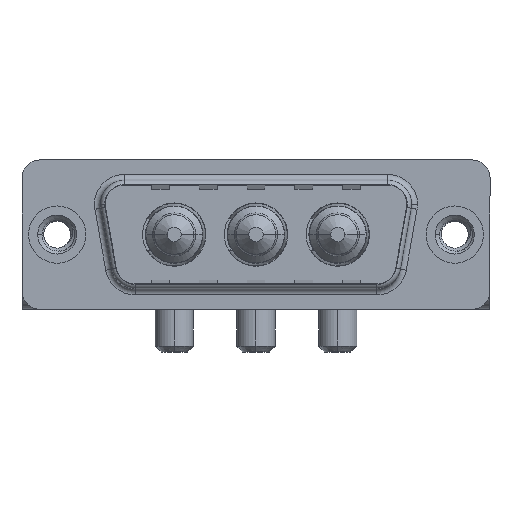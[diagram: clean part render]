
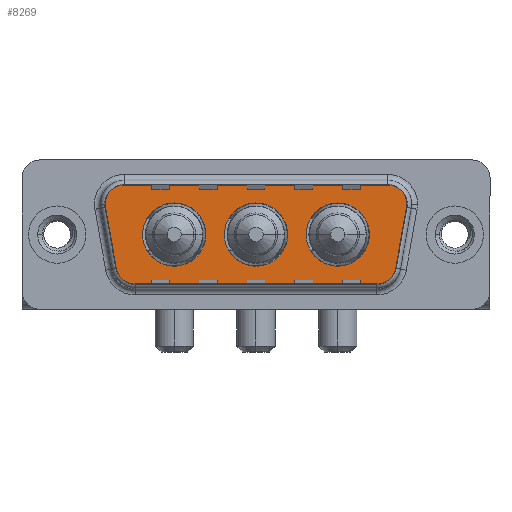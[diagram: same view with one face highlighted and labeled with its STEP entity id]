
A CAD part, top view. The second image highlights one B-rep face of the part: STEP entity #8269.
In plain terms, the highlighted planar face has unit normal (0, 0, 1).
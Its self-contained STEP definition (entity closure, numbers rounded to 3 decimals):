
#86 = VECTOR ( 'NONE', #13259, 1000. ) ;
#158 = CARTESIAN_POINT ( 'NONE',  ( 16.65, 0., 0. ) ) ;
#438 = CARTESIAN_POINT ( 'NONE',  ( 9.8, 0., 0. ) ) ;
#579 = ORIENTED_EDGE ( 'NONE', *, *, #2384, .F. ) ;
#604 = CARTESIAN_POINT ( 'NONE',  ( 5.411, 2.9, 0. ) ) ;
#606 = EDGE_CURVE ( 'NONE', #11019, #8683, #7015, .T. ) ;
#707 = ORIENTED_EDGE ( 'NONE', *, *, #3189, .T. ) ;
#709 = DIRECTION ( 'NONE',  ( 1., 0., 0. ) ) ;
#790 = DIRECTION ( 'NONE',  ( 0., 0., 1. ) ) ;
#871 = ORIENTED_EDGE ( 'NONE', *, *, #606, .T. ) ;
#988 = EDGE_CURVE ( 'NONE', #10043, #11019, #12778, .T. ) ;
#1168 = AXIS2_PLACEMENT_3D ( 'NONE', #10841, #5732, #5518 ) ;
#1506 = CARTESIAN_POINT ( 'NONE',  ( 29.889, 2.9, 0. ) ) ;
#1746 = FACE_BOUND ( 'NONE', #6988, .T. ) ;
#1797 = CARTESIAN_POINT ( 'NONE',  ( 29.859, 2.553, 0. ) ) ;
#1810 = EDGE_CURVE ( 'NONE', #2459, #10043, #4019, .T. ) ;
#1929 = VERTEX_POINT ( 'NONE', #11350 ) ;
#1930 = ORIENTED_EDGE ( 'NONE', *, *, #6689, .F. ) ;
#2007 = AXIS2_PLACEMENT_3D ( 'NONE', #6877, #3414, #4720 ) ;
#2245 = AXIS2_PLACEMENT_3D ( 'NONE', #158, #6421, #7410 ) ;
#2384 = EDGE_CURVE ( 'NONE', #12608, #10893, #13707, .T. ) ;
#2459 = VERTEX_POINT ( 'NONE', #3282 ) ;
#2910 = CIRCLE ( 'NONE', #2007, 2. ) ;
#3064 = DIRECTION ( 'NONE',  ( 0.174, -0.985, 0. ) ) ;
#3143 = EDGE_CURVE ( 'NONE', #6849, #7080, #2910, .T. ) ;
#3158 = DIRECTION ( 'NONE',  ( 0., 0., 1. ) ) ;
#3189 = EDGE_CURVE ( 'NONE', #7080, #8684, #8976, .T. ) ;
#3282 = CARTESIAN_POINT ( 'NONE',  ( 5.411, 4.9, 0. ) ) ;
#3364 = CIRCLE ( 'NONE', #13649, 2. ) ;
#3414 = DIRECTION ( 'NONE',  ( 0., 0., 1. ) ) ;
#3438 = ORIENTED_EDGE ( 'NONE', *, *, #8021, .T. ) ;
#3550 = ORIENTED_EDGE ( 'NONE', *, *, #9644, .F. ) ;
#3676 = EDGE_CURVE ( 'NONE', #13071, #8452, #9568, .T. ) ;
#3910 = VERTEX_POINT ( 'NONE', #6340 ) ;
#4019 = CIRCLE ( 'NONE', #13632, 2. ) ;
#4056 = DIRECTION ( 'NONE',  ( 0., 0., 1. ) ) ;
#4114 = CARTESIAN_POINT ( 'NONE',  ( 3.441, 2.553, 0. ) ) ;
#4203 = DIRECTION ( 'NONE',  ( -1., 0., 0. ) ) ;
#4568 = AXIS2_PLACEMENT_3D ( 'NONE', #6428, #3158, #4203 ) ;
#4661 = CARTESIAN_POINT ( 'NONE',  ( 20.85, 0., 0. ) ) ;
#4696 = DIRECTION ( 'NONE',  ( 0., 0., 1. ) ) ;
#4701 = DIRECTION ( 'NONE',  ( 1., 0., 0. ) ) ;
#4717 = CIRCLE ( 'NONE', #8948, 2.65 ) ;
#4720 = DIRECTION ( 'NONE',  ( 1., 0., 0. ) ) ;
#4723 = CIRCLE ( 'NONE', #10959, 2.65 ) ;
#4849 = EDGE_CURVE ( 'NONE', #12040, #1929, #6034, .T. ) ;
#4884 = CARTESIAN_POINT ( 'NONE',  ( 12.45, 0., 0. ) ) ;
#4943 = AXIS2_PLACEMENT_3D ( 'NONE', #6475, #9352, #13788 ) ;
#4944 = CARTESIAN_POINT ( 'NONE',  ( 6.434, -4.9, 0. ) ) ;
#5052 = DIRECTION ( 'NONE',  ( 1., 0., 0. ) ) ;
#5430 = EDGE_CURVE ( 'NONE', #8452, #13071, #13432, .T. ) ;
#5518 = DIRECTION ( 'NONE',  ( -1., 0., 0. ) ) ;
#5732 = DIRECTION ( 'NONE',  ( 0., 0., 1. ) ) ;
#5770 = DIRECTION ( 'NONE',  ( -1., 0., 0. ) ) ;
#5779 = VECTOR ( 'NONE', #8898, 1000. ) ;
#5873 = AXIS2_PLACEMENT_3D ( 'NONE', #13583, #790, #5052 ) ;
#5900 = LINE ( 'NONE', #10170, #5779 ) ;
#5956 = CARTESIAN_POINT ( 'NONE',  ( 14., 0., 0. ) ) ;
#6034 = CIRCLE ( 'NONE', #2245, 2.65 ) ;
#6064 = FACE_BOUND ( 'NONE', #9655, .T. ) ;
#6129 = CARTESIAN_POINT ( 'NONE',  ( 28.836, -3.247, 0. ) ) ;
#6251 = EDGE_CURVE ( 'NONE', #9187, #3910, #3364, .T. ) ;
#6340 = CARTESIAN_POINT ( 'NONE',  ( 27.889, 4.9, 0. ) ) ;
#6421 = DIRECTION ( 'NONE',  ( 0., 0., 1. ) ) ;
#6428 = CARTESIAN_POINT ( 'NONE',  ( 6.434, -2.9, 0. ) ) ;
#6475 = CARTESIAN_POINT ( 'NONE',  ( 23.5, 0., 0. ) ) ;
#6567 = ORIENTED_EDGE ( 'NONE', *, *, #9221, .T. ) ;
#6689 = EDGE_CURVE ( 'NONE', #1929, #12040, #4717, .T. ) ;
#6797 = DIRECTION ( 'NONE',  ( 0., 0., 1. ) ) ;
#6849 = VERTEX_POINT ( 'NONE', #10753 ) ;
#6877 = CARTESIAN_POINT ( 'NONE',  ( 26.866, -2.9, 0. ) ) ;
#6977 = CIRCLE ( 'NONE', #1168, 2. ) ;
#6988 = EDGE_LOOP ( 'NONE', ( #10766, #7136 ) ) ;
#7015 = CIRCLE ( 'NONE', #4568, 2. ) ;
#7080 = VERTEX_POINT ( 'NONE', #6129 ) ;
#7136 = ORIENTED_EDGE ( 'NONE', *, *, #5430, .F. ) ;
#7196 = AXIS2_PLACEMENT_3D ( 'NONE', #8430, #13775, #12579 ) ;
#7217 = ORIENTED_EDGE ( 'NONE', *, *, #4849, .F. ) ;
#7410 = DIRECTION ( 'NONE',  ( 1., 0., 0. ) ) ;
#7511 = ORIENTED_EDGE ( 'NONE', *, *, #3143, .T. ) ;
#7791 = DIRECTION ( 'NONE',  ( 0., 0., 1. ) ) ;
#8011 = CARTESIAN_POINT ( 'NONE',  ( 4.464, -3.247, 0. ) ) ;
#8021 = EDGE_CURVE ( 'NONE', #8684, #9187, #6977, .T. ) ;
#8026 = CARTESIAN_POINT ( 'NONE',  ( 3.441, 2.553, 0. ) ) ;
#8190 = EDGE_LOOP ( 'NONE', ( #1930, #7217 ) ) ;
#8258 = ORIENTED_EDGE ( 'NONE', *, *, #988, .T. ) ;
#8269 = ADVANCED_FACE ( 'NONE', ( #11321, #1746, #6064, #10342 ), #8373, .T. ) ;
#8373 = PLANE ( 'NONE',  #7196 ) ;
#8430 = CARTESIAN_POINT ( 'NONE',  ( 26.866, -2.9, 0. ) ) ;
#8452 = VERTEX_POINT ( 'NONE', #4661 ) ;
#8607 = CARTESIAN_POINT ( 'NONE',  ( 26.15, 0., 0. ) ) ;
#8683 = VERTEX_POINT ( 'NONE', #4944 ) ;
#8684 = VERTEX_POINT ( 'NONE', #1797 ) ;
#8887 = CARTESIAN_POINT ( 'NONE',  ( 23.5, 0., 0. ) ) ;
#8898 = DIRECTION ( 'NONE',  ( -1., 0., 0. ) ) ;
#8948 = AXIS2_PLACEMENT_3D ( 'NONE', #9151, #4056, #709 ) ;
#8952 = DIRECTION ( 'NONE',  ( 1., 0., 0. ) ) ;
#8976 = LINE ( 'NONE', #12272, #86 ) ;
#9001 = ORIENTED_EDGE ( 'NONE', *, *, #6251, .T. ) ;
#9151 = CARTESIAN_POINT ( 'NONE',  ( 16.65, 0., 0. ) ) ;
#9187 = VERTEX_POINT ( 'NONE', #1506 ) ;
#9221 = EDGE_CURVE ( 'NONE', #3910, #2459, #5900, .T. ) ;
#9352 = DIRECTION ( 'NONE',  ( 0., 0., 1. ) ) ;
#9568 = CIRCLE ( 'NONE', #10265, 2.65 ) ;
#9581 = ORIENTED_EDGE ( 'NONE', *, *, #13531, .T. ) ;
#9644 = EDGE_CURVE ( 'NONE', #10893, #12608, #4723, .T. ) ;
#9655 = EDGE_LOOP ( 'NONE', ( #3550, #579 ) ) ;
#9964 = VECTOR ( 'NONE', #3064, 1000. ) ;
#10043 = VERTEX_POINT ( 'NONE', #8026 ) ;
#10170 = CARTESIAN_POINT ( 'NONE',  ( 5.411, 4.9, 0. ) ) ;
#10182 = DIRECTION ( 'NONE',  ( 0., 0., 1. ) ) ;
#10265 = AXIS2_PLACEMENT_3D ( 'NONE', #8887, #6797, #4701 ) ;
#10342 = FACE_OUTER_BOUND ( 'NONE', #11283, .T. ) ;
#10692 = ORIENTED_EDGE ( 'NONE', *, *, #1810, .T. ) ;
#10753 = CARTESIAN_POINT ( 'NONE',  ( 26.866, -4.9, 0. ) ) ;
#10766 = ORIENTED_EDGE ( 'NONE', *, *, #3676, .F. ) ;
#10841 = CARTESIAN_POINT ( 'NONE',  ( 27.889, 2.9, 0. ) ) ;
#10893 = VERTEX_POINT ( 'NONE', #4884 ) ;
#10959 = AXIS2_PLACEMENT_3D ( 'NONE', #438, #4696, #8952 ) ;
#11019 = VERTEX_POINT ( 'NONE', #8011 ) ;
#11081 = DIRECTION ( 'NONE',  ( 1., 0., 0. ) ) ;
#11283 = EDGE_LOOP ( 'NONE', ( #7511, #707, #3438, #9001, #6567, #10692, #8258, #871, #9581 ) ) ;
#11321 = FACE_BOUND ( 'NONE', #8190, .T. ) ;
#11350 = CARTESIAN_POINT ( 'NONE',  ( 19.3, 0., 0. ) ) ;
#11459 = CARTESIAN_POINT ( 'NONE',  ( 7.15, 0., 0. ) ) ;
#11814 = DIRECTION ( 'NONE',  ( 1., 0., 0. ) ) ;
#12040 = VERTEX_POINT ( 'NONE', #5956 ) ;
#12272 = CARTESIAN_POINT ( 'NONE',  ( 29.859, 2.553, 0. ) ) ;
#12579 = DIRECTION ( 'NONE',  ( 1., 0., 0. ) ) ;
#12608 = VERTEX_POINT ( 'NONE', #11459 ) ;
#12728 = CARTESIAN_POINT ( 'NONE',  ( 6.434, -4.9, 0. ) ) ;
#12778 = LINE ( 'NONE', #4114, #9964 ) ;
#12800 = LINE ( 'NONE', #12728, #12841 ) ;
#12841 = VECTOR ( 'NONE', #11814, 1000. ) ;
#13071 = VERTEX_POINT ( 'NONE', #8607 ) ;
#13259 = DIRECTION ( 'NONE',  ( 0.174, 0.985, 0. ) ) ;
#13341 = CARTESIAN_POINT ( 'NONE',  ( 27.889, 2.9, 0. ) ) ;
#13432 = CIRCLE ( 'NONE', #4943, 2.65 ) ;
#13531 = EDGE_CURVE ( 'NONE', #8683, #6849, #12800, .T. ) ;
#13583 = CARTESIAN_POINT ( 'NONE',  ( 9.8, 0., 0. ) ) ;
#13632 = AXIS2_PLACEMENT_3D ( 'NONE', #604, #7791, #11081 ) ;
#13649 = AXIS2_PLACEMENT_3D ( 'NONE', #13341, #10182, #5770 ) ;
#13707 = CIRCLE ( 'NONE', #5873, 2.65 ) ;
#13775 = DIRECTION ( 'NONE',  ( 0., 0., 1. ) ) ;
#13788 = DIRECTION ( 'NONE',  ( 1., 0., 0. ) ) ;
